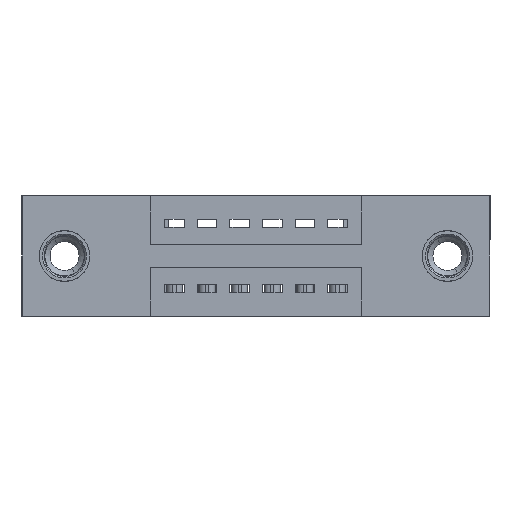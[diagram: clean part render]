
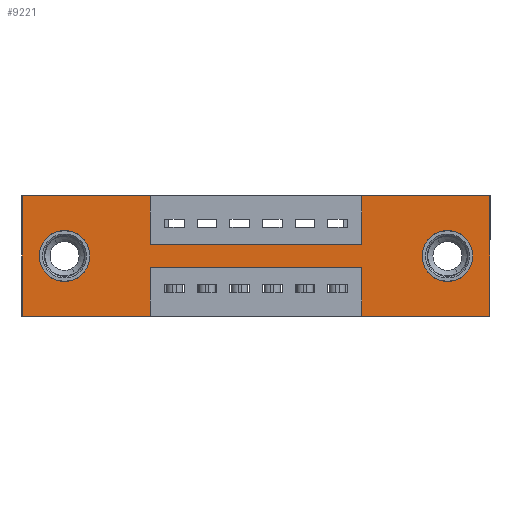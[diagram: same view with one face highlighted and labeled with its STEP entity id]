
A CAD part, front view. The second image highlights one B-rep face of the part: STEP entity #9221.
In plain terms, the highlighted planar face has unit normal (0, -1, 0).
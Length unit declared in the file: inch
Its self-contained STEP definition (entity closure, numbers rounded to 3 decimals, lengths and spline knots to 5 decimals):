
#90 = VECTOR ( 'NONE', #1156, 39.37008 ) ;
#106 = VERTEX_POINT ( 'NONE', #6540 ) ;
#119 = DIRECTION ( 'NONE',  ( 0., -1., 0. ) ) ;
#206 = CARTESIAN_POINT ( 'NONE',  ( 1.435, 0., 0. ) ) ;
#418 = AXIS2_PLACEMENT_3D ( 'NONE', #1781, #3538, #11343 ) ;
#487 = CARTESIAN_POINT ( 'NONE',  ( 1.0425, 0., -0.37 ) ) ;
#591 = CARTESIAN_POINT ( 'NONE',  ( 1.305, 0., -0.185 ) ) ;
#631 = DIRECTION ( 'NONE',  ( 0., 1., 0. ) ) ;
#728 = ORIENTED_EDGE ( 'NONE', *, *, #6776, .F. ) ;
#733 = VECTOR ( 'NONE', #11412, 39.37008 ) ;
#878 = DIRECTION ( 'NONE',  ( 0., 0., -1. ) ) ;
#969 = ORIENTED_EDGE ( 'NONE', *, *, #8229, .T. ) ;
#1003 = EDGE_CURVE ( 'NONE', #10730, #8213, #1820, .T. ) ;
#1022 = LINE ( 'NONE', #206, #7672 ) ;
#1156 = DIRECTION ( 'NONE',  ( 0., 0., -1. ) ) ;
#1166 = ORIENTED_EDGE ( 'NONE', *, *, #8989, .F. ) ;
#1295 = VECTOR ( 'NONE', #9485, 39.37008 ) ;
#1483 = CARTESIAN_POINT ( 'NONE',  ( 1.305, 0., -0.107 ) ) ;
#1586 = CARTESIAN_POINT ( 'NONE',  ( 0., 0., -0.37 ) ) ;
#1592 = CARTESIAN_POINT ( 'NONE',  ( 1.435, 0., -0.37 ) ) ;
#1627 = CARTESIAN_POINT ( 'NONE',  ( 0., 0., 0. ) ) ;
#1768 = VERTEX_POINT ( 'NONE', #7019 ) ;
#1781 = CARTESIAN_POINT ( 'NONE',  ( 0.13, 0., -0.185 ) ) ;
#1786 = DIRECTION ( 'NONE',  ( 0., 0., 1. ) ) ;
#1820 = CIRCLE ( 'NONE', #9329, 0.078 ) ;
#1881 = CARTESIAN_POINT ( 'NONE',  ( 0., 0., -0.37 ) ) ;
#1919 = DIRECTION ( 'NONE',  ( -1., 0., 0. ) ) ;
#1929 = CARTESIAN_POINT ( 'NONE',  ( 0., 0., -0.37 ) ) ;
#1980 = ORIENTED_EDGE ( 'NONE', *, *, #4469, .F. ) ;
#2139 = CARTESIAN_POINT ( 'NONE',  ( 0.3925, 0., -0.37 ) ) ;
#2227 = FACE_BOUND ( 'NONE', #2973, .T. ) ;
#2307 = VERTEX_POINT ( 'NONE', #7290 ) ;
#2319 = AXIS2_PLACEMENT_3D ( 'NONE', #3009, #4856, #11097 ) ;
#2335 = CARTESIAN_POINT ( 'NONE',  ( 0.3925, 0., -0.15 ) ) ;
#2360 = FACE_BOUND ( 'NONE', #5281, .T. ) ;
#2397 = DIRECTION ( 'NONE',  ( 0., 0., 1. ) ) ;
#2522 = VERTEX_POINT ( 'NONE', #10474 ) ;
#2912 = DIRECTION ( 'NONE',  ( 0., 0., -1. ) ) ;
#2973 = EDGE_LOOP ( 'NONE', ( #9374, #4113 ) ) ;
#3009 = CARTESIAN_POINT ( 'NONE',  ( 0.13, 0., -0.185 ) ) ;
#3137 = VECTOR ( 'NONE', #7921, 39.37008 ) ;
#3148 = CIRCLE ( 'NONE', #8767, 0.078 ) ;
#3236 = LINE ( 'NONE', #1881, #11172 ) ;
#3538 = DIRECTION ( 'NONE',  ( 0., 1., 0. ) ) ;
#3585 = ORIENTED_EDGE ( 'NONE', *, *, #5813, .F. ) ;
#3604 = VERTEX_POINT ( 'NONE', #10898 ) ;
#3617 = CARTESIAN_POINT ( 'NONE',  ( 0.3925, 0., 0. ) ) ;
#4113 = ORIENTED_EDGE ( 'NONE', *, *, #10776, .T. ) ;
#4272 = CARTESIAN_POINT ( 'NONE',  ( 0.3925, 0., -0.22 ) ) ;
#4469 = EDGE_CURVE ( 'NONE', #5761, #3604, #6275, .T. ) ;
#4486 = ORIENTED_EDGE ( 'NONE', *, *, #5083, .F. ) ;
#4533 = VERTEX_POINT ( 'NONE', #7841 ) ;
#4650 = VERTEX_POINT ( 'NONE', #3617 ) ;
#4695 = FACE_OUTER_BOUND ( 'NONE', #11196, .T. ) ;
#4730 = VERTEX_POINT ( 'NONE', #1929 ) ;
#4856 = DIRECTION ( 'NONE',  ( 0., 1., 0. ) ) ;
#5009 = DIRECTION ( 'NONE',  ( -1., 0., 0. ) ) ;
#5034 = DIRECTION ( 'NONE',  ( 1., 0., 0. ) ) ;
#5074 = CARTESIAN_POINT ( 'NONE',  ( 0.13, 0., -0.263 ) ) ;
#5083 = EDGE_CURVE ( 'NONE', #6153, #5761, #6681, .T. ) ;
#5141 = CARTESIAN_POINT ( 'NONE',  ( 0.3925, 0., -0.22 ) ) ;
#5280 = EDGE_CURVE ( 'NONE', #1768, #4730, #3236, .T. ) ;
#5281 = EDGE_LOOP ( 'NONE', ( #5393, #969 ) ) ;
#5302 = VECTOR ( 'NONE', #5009, 39.37008 ) ;
#5313 = VERTEX_POINT ( 'NONE', #9942 ) ;
#5371 = PLANE ( 'NONE',  #8960 ) ;
#5386 = CARTESIAN_POINT ( 'NONE',  ( 0., 0., 0. ) ) ;
#5389 = EDGE_CURVE ( 'NONE', #9414, #1768, #11019, .T. ) ;
#5393 = ORIENTED_EDGE ( 'NONE', *, *, #9313, .T. ) ;
#5399 = LINE ( 'NONE', #5141, #733 ) ;
#5462 = CARTESIAN_POINT ( 'NONE',  ( 1.0425, 0., 0. ) ) ;
#5761 = VERTEX_POINT ( 'NONE', #6231 ) ;
#5813 = EDGE_CURVE ( 'NONE', #2307, #6153, #1022, .T. ) ;
#5977 = LINE ( 'NONE', #1627, #1295 ) ;
#6044 = LINE ( 'NONE', #7005, #3137 ) ;
#6151 = VECTOR ( 'NONE', #2397, 39.37008 ) ;
#6153 = VERTEX_POINT ( 'NONE', #1592 ) ;
#6205 = EDGE_CURVE ( 'NONE', #4730, #2522, #5977, .T. ) ;
#6231 = CARTESIAN_POINT ( 'NONE',  ( 1.0425, 0., -0.37 ) ) ;
#6275 = LINE ( 'NONE', #487, #6151 ) ;
#6370 = CIRCLE ( 'NONE', #418, 0.078 ) ;
#6540 = CARTESIAN_POINT ( 'NONE',  ( 0.13, 0., -0.107 ) ) ;
#6665 = VERTEX_POINT ( 'NONE', #5074 ) ;
#6681 = LINE ( 'NONE', #1586, #5302 ) ;
#6708 = ORIENTED_EDGE ( 'NONE', *, *, #5389, .F. ) ;
#6719 = LINE ( 'NONE', #5462, #7722 ) ;
#6776 = EDGE_CURVE ( 'NONE', #3604, #9414, #5399, .T. ) ;
#6835 = EDGE_CURVE ( 'NONE', #4650, #9493, #10991, .T. ) ;
#6867 = CARTESIAN_POINT ( 'NONE',  ( 0.3925, 0., 0. ) ) ;
#6936 = ORIENTED_EDGE ( 'NONE', *, *, #6205, .F. ) ;
#6943 = CARTESIAN_POINT ( 'NONE',  ( 0.3925, 0., -0.15 ) ) ;
#7005 = CARTESIAN_POINT ( 'NONE',  ( 0., 0., 0. ) ) ;
#7019 = CARTESIAN_POINT ( 'NONE',  ( 0.3925, 0., -0.37 ) ) ;
#7050 = ORIENTED_EDGE ( 'NONE', *, *, #11035, .F. ) ;
#7150 = CARTESIAN_POINT ( 'NONE',  ( 0., 0., -0.37 ) ) ;
#7204 = DIRECTION ( 'NONE',  ( 1., 0., 0. ) ) ;
#7290 = CARTESIAN_POINT ( 'NONE',  ( 1.435, 0., 0. ) ) ;
#7498 = VECTOR ( 'NONE', #878, 39.37008 ) ;
#7672 = VECTOR ( 'NONE', #8077, 39.37008 ) ;
#7708 = ORIENTED_EDGE ( 'NONE', *, *, #6835, .F. ) ;
#7722 = VECTOR ( 'NONE', #1786, 39.37008 ) ;
#7828 = ORIENTED_EDGE ( 'NONE', *, *, #5280, .F. ) ;
#7841 = CARTESIAN_POINT ( 'NONE',  ( 1.0425, 0., -0.15 ) ) ;
#7921 = DIRECTION ( 'NONE',  ( 1., 0., 0. ) ) ;
#8041 = VECTOR ( 'NONE', #7204, 39.37008 ) ;
#8077 = DIRECTION ( 'NONE',  ( 0., 0., -1. ) ) ;
#8154 = CARTESIAN_POINT ( 'NONE',  ( 1.305, 0., -0.185 ) ) ;
#8213 = VERTEX_POINT ( 'NONE', #10462 ) ;
#8229 = EDGE_CURVE ( 'NONE', #6665, #106, #6370, .T. ) ;
#8633 = DIRECTION ( 'NONE',  ( 0., 0., -1. ) ) ;
#8767 = AXIS2_PLACEMENT_3D ( 'NONE', #591, #631, #8633 ) ;
#8954 = DIRECTION ( 'NONE',  ( 0., 0., -1. ) ) ;
#8960 = AXIS2_PLACEMENT_3D ( 'NONE', #7150, #119, #8954 ) ;
#8989 = EDGE_CURVE ( 'NONE', #5313, #2307, #9855, .T. ) ;
#9221 = ADVANCED_FACE ( 'NONE', ( #2227, #2360, #4695 ), #5371, .T. ) ;
#9313 = EDGE_CURVE ( 'NONE', #106, #6665, #10559, .T. ) ;
#9329 = AXIS2_PLACEMENT_3D ( 'NONE', #8154, #10805, #2912 ) ;
#9374 = ORIENTED_EDGE ( 'NONE', *, *, #1003, .T. ) ;
#9414 = VERTEX_POINT ( 'NONE', #4272 ) ;
#9485 = DIRECTION ( 'NONE',  ( 0., 0., 1. ) ) ;
#9493 = VERTEX_POINT ( 'NONE', #6943 ) ;
#9855 = LINE ( 'NONE', #5386, #8041 ) ;
#9942 = CARTESIAN_POINT ( 'NONE',  ( 1.0425, 0., 0. ) ) ;
#10007 = EDGE_CURVE ( 'NONE', #9493, #4533, #10679, .T. ) ;
#10257 = ORIENTED_EDGE ( 'NONE', *, *, #10866, .F. ) ;
#10462 = CARTESIAN_POINT ( 'NONE',  ( 1.305, 0., -0.263 ) ) ;
#10474 = CARTESIAN_POINT ( 'NONE',  ( 0., 0., 0. ) ) ;
#10559 = CIRCLE ( 'NONE', #2319, 0.078 ) ;
#10679 = LINE ( 'NONE', #2335, #11238 ) ;
#10712 = ORIENTED_EDGE ( 'NONE', *, *, #10007, .F. ) ;
#10730 = VERTEX_POINT ( 'NONE', #1483 ) ;
#10776 = EDGE_CURVE ( 'NONE', #8213, #10730, #3148, .T. ) ;
#10805 = DIRECTION ( 'NONE',  ( 0., 1., 0. ) ) ;
#10866 = EDGE_CURVE ( 'NONE', #2522, #4650, #6044, .T. ) ;
#10898 = CARTESIAN_POINT ( 'NONE',  ( 1.0425, 0., -0.22 ) ) ;
#10991 = LINE ( 'NONE', #6867, #7498 ) ;
#11019 = LINE ( 'NONE', #2139, #90 ) ;
#11035 = EDGE_CURVE ( 'NONE', #4533, #5313, #6719, .T. ) ;
#11097 = DIRECTION ( 'NONE',  ( 0., 0., 1. ) ) ;
#11172 = VECTOR ( 'NONE', #1919, 39.37008 ) ;
#11196 = EDGE_LOOP ( 'NONE', ( #6708, #728, #1980, #4486, #3585, #1166, #7050, #10712, #7708, #10257, #6936, #7828 ) ) ;
#11238 = VECTOR ( 'NONE', #5034, 39.37008 ) ;
#11343 = DIRECTION ( 'NONE',  ( 0., 0., 1. ) ) ;
#11412 = DIRECTION ( 'NONE',  ( -1., 0., 0. ) ) ;
